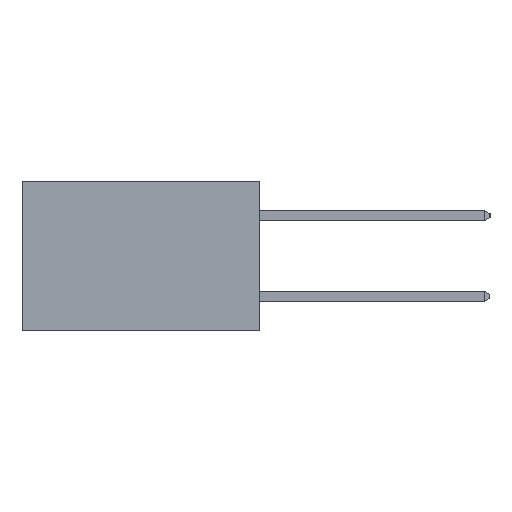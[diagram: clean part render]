
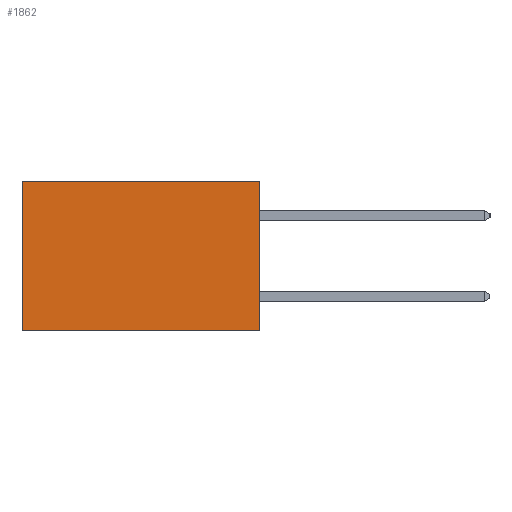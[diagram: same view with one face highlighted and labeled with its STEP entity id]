
A CAD part, left-side view. The second image highlights one B-rep face of the part: STEP entity #1862.
In plain terms, the highlighted planar face has unit normal (-1, 0, 0).
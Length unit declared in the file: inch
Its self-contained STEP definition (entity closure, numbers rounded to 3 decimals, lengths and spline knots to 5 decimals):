
#187 = ORIENTED_EDGE ( 'NONE', *, *, #918, .F. ) ;
#401 = ORIENTED_EDGE ( 'NONE', *, *, #2443, .T. ) ;
#843 = VERTEX_POINT ( 'NONE', #16398 ) ;
#918 = EDGE_CURVE ( 'NONE', #1446, #5990, #9718, .T. ) ;
#1446 = VERTEX_POINT ( 'NONE', #9814 ) ;
#1843 = VECTOR ( 'NONE', #15417, 39.37008 ) ;
#1862 = ADVANCED_FACE ( 'NONE', ( #14070 ), #11113, .F. ) ;
#2181 = EDGE_CURVE ( 'NONE', #12859, #1446, #5850, .T. ) ;
#2443 = EDGE_CURVE ( 'NONE', #12859, #843, #4375, .T. ) ;
#2685 = CARTESIAN_POINT ( 'NONE',  ( 0.277, 0.59, -0.37 ) ) ;
#2977 = ORIENTED_EDGE ( 'NONE', *, *, #2181, .F. ) ;
#3302 = DIRECTION ( 'NONE',  ( 0., 0., -1. ) ) ;
#3501 = DIRECTION ( 'NONE',  ( 1., 0., 0. ) ) ;
#4375 = LINE ( 'NONE', #13884, #8824 ) ;
#4823 = AXIS2_PLACEMENT_3D ( 'NONE', #10494, #3501, #3302 ) ;
#5850 = LINE ( 'NONE', #6595, #1843 ) ;
#5990 = VERTEX_POINT ( 'NONE', #2685 ) ;
#6444 = DIRECTION ( 'NONE',  ( 0., 0., -1. ) ) ;
#6595 = CARTESIAN_POINT ( 'NONE',  ( 0.277, 0., -0.37 ) ) ;
#8688 = ORIENTED_EDGE ( 'NONE', *, *, #10373, .T. ) ;
#8824 = VECTOR ( 'NONE', #13871, 39.37008 ) ;
#9310 = VECTOR ( 'NONE', #12021, 39.37008 ) ;
#9718 = LINE ( 'NONE', #12250, #9310 ) ;
#9814 = CARTESIAN_POINT ( 'NONE',  ( 0.277, 0., -0.37 ) ) ;
#10236 = VECTOR ( 'NONE', #6444, 39.37008 ) ;
#10373 = EDGE_CURVE ( 'NONE', #843, #5990, #14183, .T. ) ;
#10494 = CARTESIAN_POINT ( 'NONE',  ( 0.277, 0., -0.37 ) ) ;
#11113 = PLANE ( 'NONE',  #4823 ) ;
#11410 = EDGE_LOOP ( 'NONE', ( #8688, #187, #2977, #401 ) ) ;
#12021 = DIRECTION ( 'NONE',  ( 0., 1., 0. ) ) ;
#12250 = CARTESIAN_POINT ( 'NONE',  ( 0.277, 0., -0.37 ) ) ;
#12859 = VERTEX_POINT ( 'NONE', #14614 ) ;
#13224 = CARTESIAN_POINT ( 'NONE',  ( 0.277, 0.59, -0.37 ) ) ;
#13871 = DIRECTION ( 'NONE',  ( 0., 1., 0. ) ) ;
#13884 = CARTESIAN_POINT ( 'NONE',  ( 0.277, 0., 0. ) ) ;
#14070 = FACE_OUTER_BOUND ( 'NONE', #11410, .T. ) ;
#14183 = LINE ( 'NONE', #13224, #10236 ) ;
#14614 = CARTESIAN_POINT ( 'NONE',  ( 0.277, 0., 0. ) ) ;
#15417 = DIRECTION ( 'NONE',  ( 0., 0., -1. ) ) ;
#16398 = CARTESIAN_POINT ( 'NONE',  ( 0.277, 0.59, 0. ) ) ;
